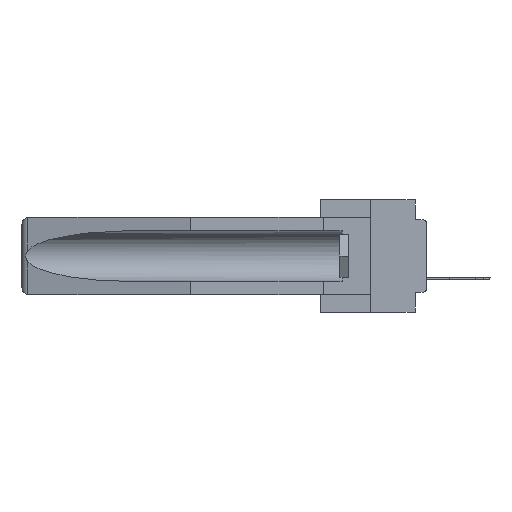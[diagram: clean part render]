
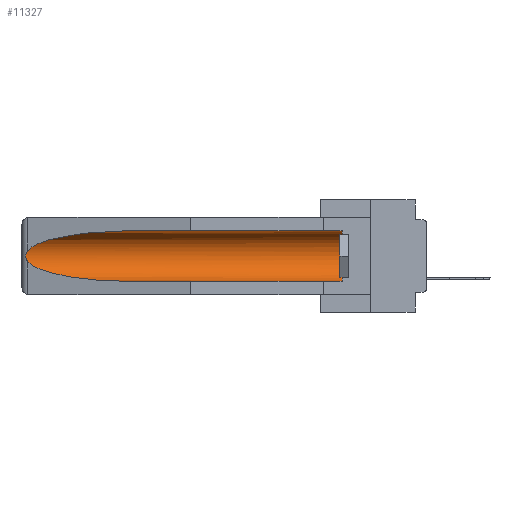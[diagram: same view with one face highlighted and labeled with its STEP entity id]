
A CAD part, left-side view. The second image highlights one B-rep face of the part: STEP entity #11327.
In plain terms, the highlighted cylindrical face has radius 2.857 mm (diameter 5.715 mm), a partial arc.
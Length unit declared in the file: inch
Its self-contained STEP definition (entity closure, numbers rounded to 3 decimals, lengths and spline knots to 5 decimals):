
#2566 = CARTESIAN_POINT ( 'NONE',  ( 0.26597, 1.52961, -0.15275 ) ) ;
#2678 = EDGE_CURVE ( 'NONE', #17435, #31699, #24484, .T. ) ;
#3084 = EDGE_CURVE ( 'NONE', #7636, #17435, #19786, .T. ) ;
#3610 = CARTESIAN_POINT ( 'NONE',  ( 0.155, 1.07973, -0.284 ) ) ;
#3882 = CARTESIAN_POINT ( 'NONE',  ( 0.155, -0.30754, -0.284 ) ) ;
#4465 = CARTESIAN_POINT ( 'NONE',  ( 0.155, 0.126, -0.1715 ) ) ;
#5699 = CARTESIAN_POINT ( 'NONE',  ( 0.26597, 1.5296, -0.19026 ) ) ;
#6270 = CARTESIAN_POINT ( 'NONE',  ( 0.26537, 1.52718, -0.14972 ) ) ;
#6463 = CARTESIAN_POINT ( 'NONE',  ( 0.26537, 1.52718, -0.14972 ) ) ;
#6525 = DIRECTION ( 'NONE',  ( 0., 0., 1. ) ) ;
#7636 = VERTEX_POINT ( 'NONE', #12565 ) ;
#8002 = ORIENTED_EDGE ( 'NONE', *, *, #34327, .T. ) ;
#8301 = EDGE_CURVE ( 'NONE', #31699, #33893, #26080, .T. ) ;
#8542 = CARTESIAN_POINT ( 'NONE',  ( 0.2673, 1.53269, -0.17917 ) ) ;
#8826 = ORIENTED_EDGE ( 'NONE', *, *, #3084, .T. ) ;
#9351 = FACE_OUTER_BOUND ( 'NONE', #16766, .T. ) ;
#10563 = CARTESIAN_POINT ( 'NONE',  ( 0.26537, 1.52718, -0.19328 ) ) ;
#10975 = CARTESIAN_POINT ( 'NONE',  ( 0.155, 0.126, -0.284 ) ) ;
#11007 = EDGE_CURVE ( 'NONE', #18343, #30183, #23543, .T. ) ;
#11290 = VECTOR ( 'NONE', #23174, 39.37008 ) ;
#11327 = ADVANCED_FACE ( 'NONE', ( #9351 ), #14603, .F. ) ;
#12474 = AXIS2_PLACEMENT_3D ( 'NONE', #4465, #32919, #32729 ) ;
#12565 = CARTESIAN_POINT ( 'NONE',  ( 0.155, 0.126, -0.059 ) ) ;
#12932 = ORIENTED_EDGE ( 'NONE', *, *, #8301, .T. ) ;
#13639 = ORIENTED_EDGE ( 'NONE', *, *, #2678, .T. ) ;
#14152 = CARTESIAN_POINT ( 'NONE',  ( 0.2675, 1.53308, -0.17534 ) ) ;
#14333 = CARTESIAN_POINT ( 'NONE',  ( 0.26654, 1.53092, -0.15636 ) ) ;
#14603 = CYLINDRICAL_SURFACE ( 'NONE', #28675, 0.1125 ) ;
#16766 = EDGE_LOOP ( 'NONE', ( #13639, #12932, #31880, #36607, #8002, #8826 ) ) ;
#17435 = VERTEX_POINT ( 'NONE', #23806 ) ;
#18343 = VERTEX_POINT ( 'NONE', #10975 ) ;
#19786 = LINE ( 'NONE', #36816, #23974 ) ;
#22249 = DIRECTION ( 'NONE',  ( 0., 1., 0. ) ) ;
#22782 = CARTESIAN_POINT ( 'NONE',  ( 0.25451, 1.48313, -0.09465 ) ) ;
#23174 = DIRECTION ( 'NONE',  ( 0., 1., 0. ) ) ;
#23490 = CARTESIAN_POINT ( 'NONE',  ( 0.26537, 1.52718, -0.19328 ) ) ;
#23543 = LINE ( 'NONE', #3882, #11290 ) ;
#23806 = CARTESIAN_POINT ( 'NONE',  ( 0.155, 1.07973, -0.059 ) ) ;
#23974 = VECTOR ( 'NONE', #22249, 39.37008 ) ;
#24484 =( BOUNDED_CURVE ( )  B_SPLINE_CURVE ( 3, ( #36811, #28941, #22782, #6270 ),
 .UNSPECIFIED., .F., .F. ) 
 B_SPLINE_CURVE_WITH_KNOTS ( ( 4, 4 ),
 ( 4.71239, 6.08839 ),
 .UNSPECIFIED. ) 
 CURVE ( )  GEOMETRIC_REPRESENTATION_ITEM ( )  RATIONAL_B_SPLINE_CURVE ( ( 1., 0.848, 0.848, 1. ) ) 
 REPRESENTATION_ITEM ( '' )  );
#24806 = CARTESIAN_POINT ( 'NONE',  ( 0.21114, 1.30732, -0.284 ) ) ;
#25054 = CIRCLE ( 'NONE', #12474, 0.1125 ) ;
#25380 = CARTESIAN_POINT ( 'NONE',  ( 0.2673, 1.5327, -0.16383 ) ) ;
#26080 = B_SPLINE_CURVE_WITH_KNOTS ( 'NONE', 3,
 ( #28370, #2566, #14333, #25380, #36789, #14152, #8542, #31350, #5699, #23490 ),
 .UNSPECIFIED., .F., .F.,
 ( 4, 2, 2, 2, 4 ),
 ( 0., 0.00029, 0.00058, 0.00087, 0.00117 ),
 .UNSPECIFIED. ) ;
#26190 = DIRECTION ( 'NONE',  ( 0., 1., 0. ) ) ;
#27322 =( BOUNDED_CURVE ( )  B_SPLINE_CURVE ( 3, ( #10563, #30775, #24806, #33761 ),
 .UNSPECIFIED., .F., .F. ) 
 B_SPLINE_CURVE_WITH_KNOTS ( ( 4, 4 ),
 ( 0.1948, 1.5708 ),
 .UNSPECIFIED. ) 
 CURVE ( )  GEOMETRIC_REPRESENTATION_ITEM ( )  RATIONAL_B_SPLINE_CURVE ( ( 1., 0.848, 0.848, 1. ) ) 
 REPRESENTATION_ITEM ( '' )  );
#27347 = CARTESIAN_POINT ( 'NONE',  ( 0.26537, 1.52718, -0.19328 ) ) ;
#28370 = CARTESIAN_POINT ( 'NONE',  ( 0.26537, 1.52718, -0.14972 ) ) ;
#28675 = AXIS2_PLACEMENT_3D ( 'NONE', #29011, #26190, #6525 ) ;
#28941 = CARTESIAN_POINT ( 'NONE',  ( 0.21114, 1.30732, -0.059 ) ) ;
#29011 = CARTESIAN_POINT ( 'NONE',  ( 0.155, -0.30754, -0.1715 ) ) ;
#30183 = VERTEX_POINT ( 'NONE', #3610 ) ;
#30775 = CARTESIAN_POINT ( 'NONE',  ( 0.25451, 1.48313, -0.24835 ) ) ;
#31350 = CARTESIAN_POINT ( 'NONE',  ( 0.26655, 1.53094, -0.18657 ) ) ;
#31699 = VERTEX_POINT ( 'NONE', #6463 ) ;
#31880 = ORIENTED_EDGE ( 'NONE', *, *, #35760, .T. ) ;
#32729 = DIRECTION ( 'NONE',  ( 0., 0., 1. ) ) ;
#32919 = DIRECTION ( 'NONE',  ( 0., -1., 0. ) ) ;
#33761 = CARTESIAN_POINT ( 'NONE',  ( 0.155, 1.07973, -0.284 ) ) ;
#33893 = VERTEX_POINT ( 'NONE', #27347 ) ;
#34327 = EDGE_CURVE ( 'NONE', #18343, #7636, #25054, .T. ) ;
#35760 = EDGE_CURVE ( 'NONE', #33893, #30183, #27322, .T. ) ;
#36607 = ORIENTED_EDGE ( 'NONE', *, *, #11007, .F. ) ;
#36789 = CARTESIAN_POINT ( 'NONE',  ( 0.2675, 1.53308, -0.16763 ) ) ;
#36811 = CARTESIAN_POINT ( 'NONE',  ( 0.155, 1.07973, -0.059 ) ) ;
#36816 = CARTESIAN_POINT ( 'NONE',  ( 0.155, -0.30754, -0.059 ) ) ;
